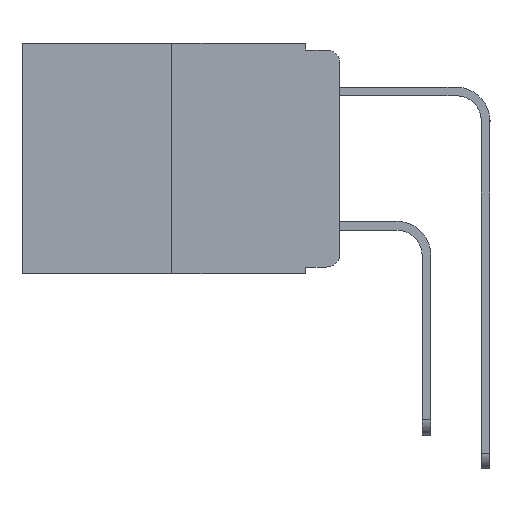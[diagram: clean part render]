
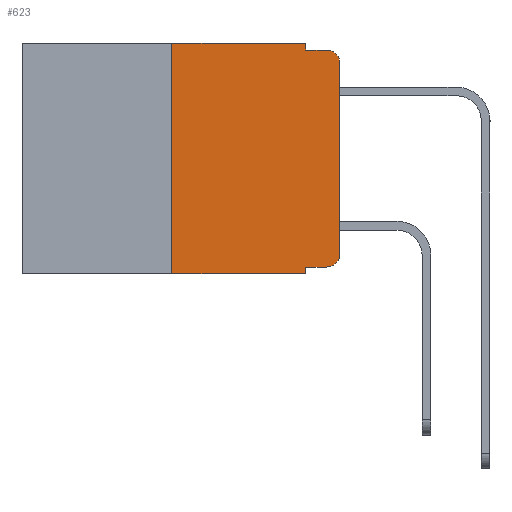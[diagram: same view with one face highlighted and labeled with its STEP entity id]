
A CAD part, left-side view. The second image highlights one B-rep face of the part: STEP entity #623.
In plain terms, the highlighted planar face has unit normal (-1, 0, 0).
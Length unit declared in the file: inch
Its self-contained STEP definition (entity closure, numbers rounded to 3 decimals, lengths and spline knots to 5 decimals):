
#133 = ORIENTED_EDGE ( 'NONE', *, *, #16002, .F. ) ;
#217 = ORIENTED_EDGE ( 'NONE', *, *, #8417, .T. ) ;
#623 = ADVANCED_FACE ( 'NONE', ( #17701 ), #20226, .F. ) ;
#737 = EDGE_CURVE ( 'NONE', #15643, #15624, #17952, .T. ) ;
#788 = CARTESIAN_POINT ( 'NONE',  ( 0., 0.051, 0. ) ) ;
#989 = LINE ( 'NONE', #19710, #9519 ) ;
#1455 = VERTEX_POINT ( 'NONE', #788 ) ;
#1506 = VERTEX_POINT ( 'NONE', #8986 ) ;
#1599 = DIRECTION ( 'NONE',  ( 0., 0., -1. ) ) ;
#2484 = DIRECTION ( 'NONE',  ( 0., 0., -1. ) ) ;
#3064 = EDGE_CURVE ( 'NONE', #15624, #4930, #11504, .T. ) ;
#3176 = CARTESIAN_POINT ( 'NONE',  ( 0., 0.02, -0.01 ) ) ;
#3385 = VERTEX_POINT ( 'NONE', #12334 ) ;
#4009 = VECTOR ( 'NONE', #18336, 39.37008 ) ;
#4125 = VERTEX_POINT ( 'NONE', #22992 ) ;
#4308 = EDGE_CURVE ( 'NONE', #9191, #3385, #14702, .T. ) ;
#4342 = LINE ( 'NONE', #16443, #18085 ) ;
#4552 = EDGE_CURVE ( 'NONE', #1506, #1455, #4342, .T. ) ;
#4930 = VERTEX_POINT ( 'NONE', #3176 ) ;
#4966 = LINE ( 'NONE', #17785, #13371 ) ;
#5577 = DIRECTION ( 'NONE',  ( -1., 0., 0. ) ) ;
#6111 = CARTESIAN_POINT ( 'NONE',  ( 0., 0.25, -0.343 ) ) ;
#6136 = ORIENTED_EDGE ( 'NONE', *, *, #4308, .F. ) ;
#6251 = CARTESIAN_POINT ( 'NONE',  ( 0., 0., -0.03 ) ) ;
#6592 = DIRECTION ( 'NONE',  ( 0., 0., -1. ) ) ;
#6622 = DIRECTION ( 'NONE',  ( 0., -1., 0. ) ) ;
#6642 = EDGE_CURVE ( 'NONE', #4125, #15643, #8778, .T. ) ;
#7627 = AXIS2_PLACEMENT_3D ( 'NONE', #18086, #5577, #20877 ) ;
#8170 = CARTESIAN_POINT ( 'NONE',  ( 0., 0., -0.313 ) ) ;
#8417 = EDGE_CURVE ( 'NONE', #22501, #3385, #20162, .T. ) ;
#8433 = CARTESIAN_POINT ( 'NONE',  ( 0., 0.02, -0.03 ) ) ;
#8591 = CARTESIAN_POINT ( 'NONE',  ( 0., 0., 0. ) ) ;
#8778 = CIRCLE ( 'NONE', #7627, 0.02 ) ;
#8920 = DIRECTION ( 'NONE',  ( 0., -1., 0. ) ) ;
#8986 = CARTESIAN_POINT ( 'NONE',  ( 0., 0.25, 0. ) ) ;
#9191 = VERTEX_POINT ( 'NONE', #15929 ) ;
#9519 = VECTOR ( 'NONE', #10922, 39.37008 ) ;
#9752 = AXIS2_PLACEMENT_3D ( 'NONE', #20482, #19959, #19955 ) ;
#10128 = ORIENTED_EDGE ( 'NONE', *, *, #18302, .F. ) ;
#10361 = DIRECTION ( 'NONE',  ( 0., -1., 0. ) ) ;
#10746 = EDGE_CURVE ( 'NONE', #1455, #20081, #22983, .T. ) ;
#10922 = DIRECTION ( 'NONE',  ( 0., 0., 1. ) ) ;
#11352 = ORIENTED_EDGE ( 'NONE', *, *, #737, .T. ) ;
#11504 = CIRCLE ( 'NONE', #22317, 0.02 ) ;
#11696 = ORIENTED_EDGE ( 'NONE', *, *, #16296, .T. ) ;
#11802 = DIRECTION ( 'NONE',  ( 0., 0., 1. ) ) ;
#12334 = CARTESIAN_POINT ( 'NONE',  ( 0., 0.051, -0.343 ) ) ;
#13047 = ORIENTED_EDGE ( 'NONE', *, *, #6642, .T. ) ;
#13213 = VECTOR ( 'NONE', #11802, 39.37008 ) ;
#13371 = VECTOR ( 'NONE', #8920, 39.37008 ) ;
#14702 = LINE ( 'NONE', #21620, #17799 ) ;
#14865 = VECTOR ( 'NONE', #6622, 39.37008 ) ;
#15624 = VERTEX_POINT ( 'NONE', #6251 ) ;
#15643 = VERTEX_POINT ( 'NONE', #8170 ) ;
#15929 = CARTESIAN_POINT ( 'NONE',  ( 0., 0.051, -0.333 ) ) ;
#16002 = EDGE_CURVE ( 'NONE', #22501, #1506, #989, .T. ) ;
#16296 = EDGE_CURVE ( 'NONE', #9191, #4125, #4966, .T. ) ;
#16341 = LINE ( 'NONE', #18265, #4009 ) ;
#16443 = CARTESIAN_POINT ( 'NONE',  ( 0., 0.473, 0. ) ) ;
#17278 = ORIENTED_EDGE ( 'NONE', *, *, #10746, .F. ) ;
#17701 = FACE_OUTER_BOUND ( 'NONE', #21112, .T. ) ;
#17785 = CARTESIAN_POINT ( 'NONE',  ( 0., 0.051, -0.333 ) ) ;
#17799 = VECTOR ( 'NONE', #1599, 39.37008 ) ;
#17952 = LINE ( 'NONE', #8591, #13213 ) ;
#18085 = VECTOR ( 'NONE', #10361, 39.37008 ) ;
#18086 = CARTESIAN_POINT ( 'NONE',  ( 0., 0.02, -0.313 ) ) ;
#18265 = CARTESIAN_POINT ( 'NONE',  ( 0., 0.051, -0.01 ) ) ;
#18302 = EDGE_CURVE ( 'NONE', #20081, #4930, #16341, .T. ) ;
#18336 = DIRECTION ( 'NONE',  ( 0., -1., 0. ) ) ;
#18424 = VECTOR ( 'NONE', #2484, 39.37008 ) ;
#18621 = CARTESIAN_POINT ( 'NONE',  ( 0., 0.051, 0. ) ) ;
#19056 = DIRECTION ( 'NONE',  ( -1., 0., 0. ) ) ;
#19090 = CARTESIAN_POINT ( 'NONE',  ( 0., 0.473, -0.343 ) ) ;
#19592 = ORIENTED_EDGE ( 'NONE', *, *, #3064, .T. ) ;
#19710 = CARTESIAN_POINT ( 'NONE',  ( 0., 0.25, 0. ) ) ;
#19955 = DIRECTION ( 'NONE',  ( 0., 0., -1. ) ) ;
#19959 = DIRECTION ( 'NONE',  ( 1., 0., 0. ) ) ;
#20081 = VERTEX_POINT ( 'NONE', #22417 ) ;
#20162 = LINE ( 'NONE', #19090, #14865 ) ;
#20226 = PLANE ( 'NONE',  #9752 ) ;
#20482 = CARTESIAN_POINT ( 'NONE',  ( 0., 0.473, 0. ) ) ;
#20877 = DIRECTION ( 'NONE',  ( 0., 0., -1. ) ) ;
#21112 = EDGE_LOOP ( 'NONE', ( #11352, #19592, #10128, #17278, #23078, #133, #217, #6136, #11696, #13047 ) ) ;
#21620 = CARTESIAN_POINT ( 'NONE',  ( 0., 0.051, 0. ) ) ;
#22317 = AXIS2_PLACEMENT_3D ( 'NONE', #8433, #19056, #6592 ) ;
#22417 = CARTESIAN_POINT ( 'NONE',  ( 0., 0.051, -0.01 ) ) ;
#22501 = VERTEX_POINT ( 'NONE', #6111 ) ;
#22983 = LINE ( 'NONE', #18621, #18424 ) ;
#22992 = CARTESIAN_POINT ( 'NONE',  ( 0., 0.02, -0.333 ) ) ;
#23078 = ORIENTED_EDGE ( 'NONE', *, *, #4552, .F. ) ;
